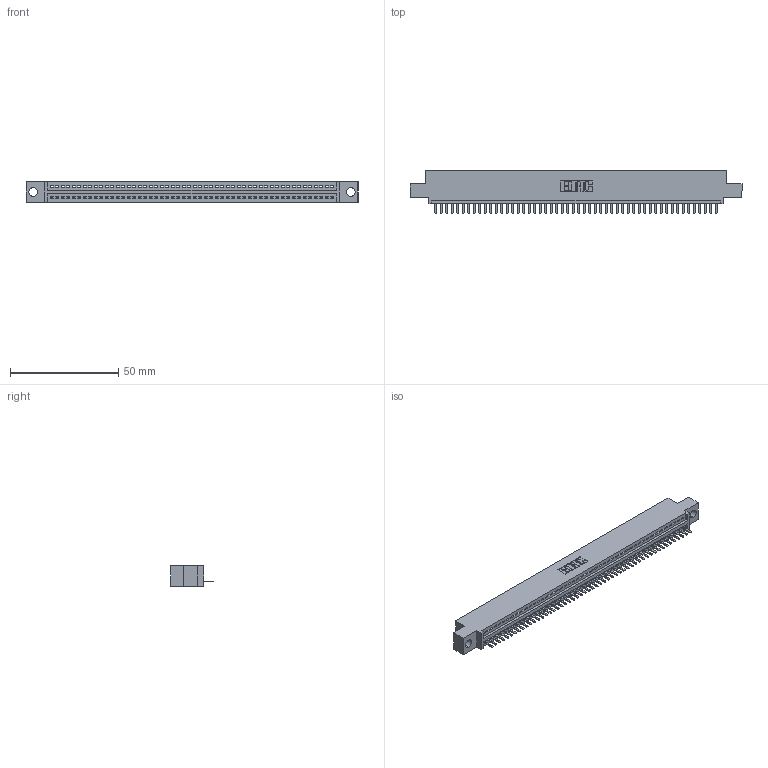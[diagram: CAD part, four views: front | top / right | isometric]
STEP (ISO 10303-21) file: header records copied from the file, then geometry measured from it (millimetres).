
FILE_DESCRIPTION (( 'STEP AP203' ), '1' );
FILE_NAME ('395-052-520-404.STEP', '2018-11-20T20:44:04', ( '' ), ( '' ), 'SwSTEP 2.0', 'SolidWorks 2016', '' );
FILE_SCHEMA (( 'CONFIG_CONTROL_DESIGN' ));
Length unit declared in the file: inch
Products named in the file (3): 395-052-520-404; 345-292-001_345-293-120; 345 Part_0.110 Offset - 0.156 Dia-TH
Assembly tree (53 placements, depth 2):
  395-052-520-404
    345 Part_0.110 Offset - 0.156 Dia-TH
    345-292-001_345-293-120  x52
Bounding box: 153.29 x 19.68 x 9.4 mm (x, y, z)
Volume: 14330.7 mm3; surface area: 18581.4 mm2
Topology: 53 solids, 53 shells, 3354 faces, 9921 edges, 6474 vertices
Faces by surface type: plane 2268, cylinder 1086
Entity records: 38039 total; most frequent: CARTESIAN_POINT 6608, ORIENTED_EDGE 6582, DIRECTION 5743, EDGE_CURVE 3291, LINE 2947, VECTOR 2947, VERTEX_POINT 2190, AXIS2_PLACEMENT_3D 1398
